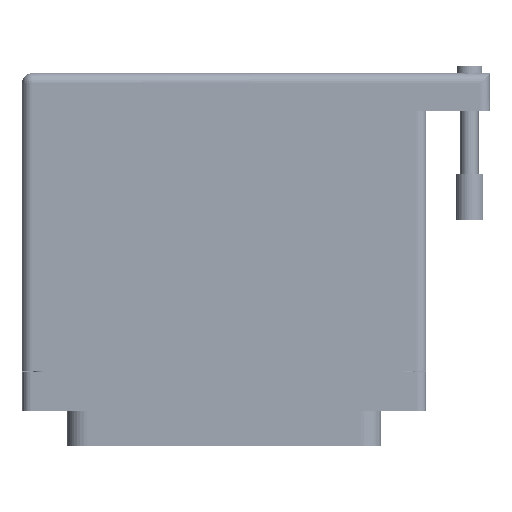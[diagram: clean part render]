
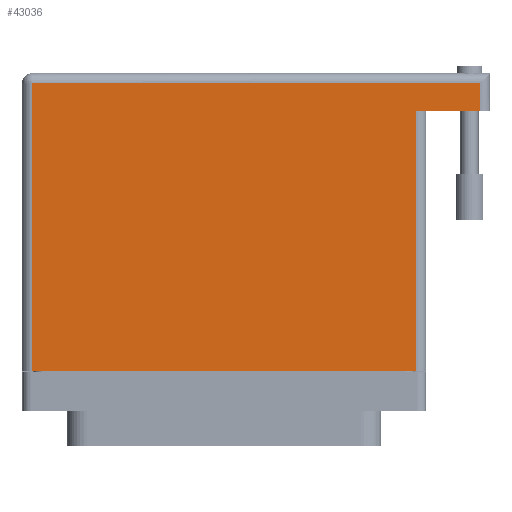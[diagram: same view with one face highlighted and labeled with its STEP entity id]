
A CAD part, front view. The second image highlights one B-rep face of the part: STEP entity #43036.
In plain terms, the highlighted face is planar.
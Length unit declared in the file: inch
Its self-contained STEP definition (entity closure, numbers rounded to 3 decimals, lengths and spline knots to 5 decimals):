
#729 = VECTOR ( 'NONE', #6900, 39.37008 ) ;
#4548 = DIRECTION ( 'NONE',  ( 0., 1., 0. ) ) ;
#5099 = CARTESIAN_POINT ( 'NONE',  ( 1.7425, 1.93, 0.765 ) ) ;
#5376 = CARTESIAN_POINT ( 'NONE',  ( -1.3775, 1.86, 0.765 ) ) ;
#6900 = DIRECTION ( 'NONE',  ( 1., 0., 0. ) ) ;
#8012 = LINE ( 'NONE', #5099, #43668 ) ;
#8445 = EDGE_CURVE ( 'NONE', #87822, #68814, #47408, .T. ) ;
#8598 = VECTOR ( 'NONE', #73439, 39.37008 ) ;
#9330 = EDGE_CURVE ( 'NONE', #84353, #87822, #8012, .T. ) ;
#9525 = EDGE_CURVE ( 'NONE', #49090, #31358, #28491, .T. ) ;
#10476 = AXIS2_PLACEMENT_3D ( 'NONE', #46919, #33085, #88435 ) ;
#12719 = ORIENTED_EDGE ( 'NONE', *, *, #35812, .T. ) ;
#12969 = ORIENTED_EDGE ( 'NONE', *, *, #9525, .T. ) ;
#17084 = ORIENTED_EDGE ( 'NONE', *, *, #9330, .T. ) ;
#18856 = CARTESIAN_POINT ( 'NONE',  ( -1.3075, -0.1, 0.765 ) ) ;
#22213 = LINE ( 'NONE', #60172, #729 ) ;
#27625 = VECTOR ( 'NONE', #55761, 39.37008 ) ;
#28491 = LINE ( 'NONE', #63098, #62875 ) ;
#31358 = VERTEX_POINT ( 'NONE', #43116 ) ;
#33085 = DIRECTION ( 'NONE',  ( 0., 0., -1. ) ) ;
#35812 = EDGE_CURVE ( 'NONE', #83724, #49090, #22213, .T. ) ;
#36090 = DIRECTION ( 'NONE',  ( 0., -1., 0. ) ) ;
#36869 = CARTESIAN_POINT ( 'NONE',  ( 1.7425, 1.86, 0.765 ) ) ;
#39126 = LINE ( 'NONE', #85143, #67114 ) ;
#40459 = LINE ( 'NONE', #69046, #27625 ) ;
#43036 = ADVANCED_FACE ( 'NONE', ( #78784 ), #60145, .F. ) ;
#43116 = CARTESIAN_POINT ( 'NONE',  ( 1.3075, 1.674, 0.765 ) ) ;
#43668 = VECTOR ( 'NONE', #4548, 39.37008 ) ;
#45591 = CARTESIAN_POINT ( 'NONE',  ( 1.3075, -0.1, 0.765 ) ) ;
#46919 = CARTESIAN_POINT ( 'NONE',  ( -1.3775, 1.93, 0.765 ) ) ;
#47408 = LINE ( 'NONE', #5376, #8598 ) ;
#49090 = VERTEX_POINT ( 'NONE', #45591 ) ;
#55761 = DIRECTION ( 'NONE',  ( -1., 0., 0. ) ) ;
#60145 = PLANE ( 'NONE',  #10476 ) ;
#60172 = CARTESIAN_POINT ( 'NONE',  ( -1.3775, -0.1, 0.765 ) ) ;
#62832 = ORIENTED_EDGE ( 'NONE', *, *, #65270, .T. ) ;
#62875 = VECTOR ( 'NONE', #82453, 39.37008 ) ;
#63098 = CARTESIAN_POINT ( 'NONE',  ( 1.3075, 1.674, 0.765 ) ) ;
#65270 = EDGE_CURVE ( 'NONE', #68814, #83724, #39126, .T. ) ;
#66152 = EDGE_LOOP ( 'NONE', ( #12719, #12969, #81547, #17084, #67696, #62832 ) ) ;
#67114 = VECTOR ( 'NONE', #36090, 39.37008 ) ;
#67696 = ORIENTED_EDGE ( 'NONE', *, *, #8445, .T. ) ;
#68814 = VERTEX_POINT ( 'NONE', #88326 ) ;
#69046 = CARTESIAN_POINT ( 'NONE',  ( 1.8125, 1.674, 0.765 ) ) ;
#71708 = CARTESIAN_POINT ( 'NONE',  ( 1.7425, 1.674, 0.765 ) ) ;
#73439 = DIRECTION ( 'NONE',  ( -1., 0., 0. ) ) ;
#78475 = EDGE_CURVE ( 'NONE', #84353, #31358, #40459, .T. ) ;
#78784 = FACE_OUTER_BOUND ( 'NONE', #66152, .T. ) ;
#81547 = ORIENTED_EDGE ( 'NONE', *, *, #78475, .F. ) ;
#82453 = DIRECTION ( 'NONE',  ( 0., 1., 0. ) ) ;
#83724 = VERTEX_POINT ( 'NONE', #18856 ) ;
#84353 = VERTEX_POINT ( 'NONE', #71708 ) ;
#85143 = CARTESIAN_POINT ( 'NONE',  ( -1.3075, -0.1, 0.765 ) ) ;
#87822 = VERTEX_POINT ( 'NONE', #36869 ) ;
#88326 = CARTESIAN_POINT ( 'NONE',  ( -1.3075, 1.86, 0.765 ) ) ;
#88435 = DIRECTION ( 'NONE',  ( -1., 0., 0. ) ) ;
